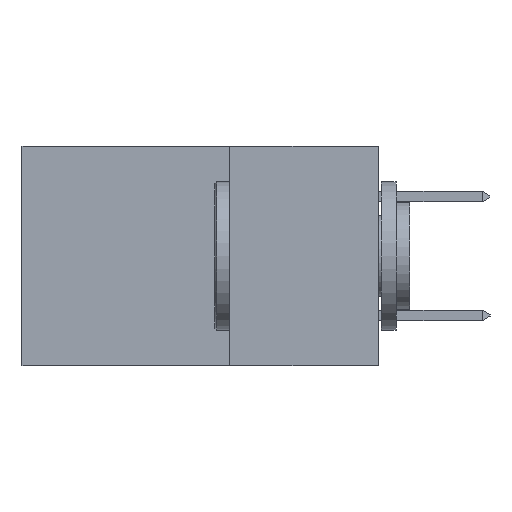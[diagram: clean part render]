
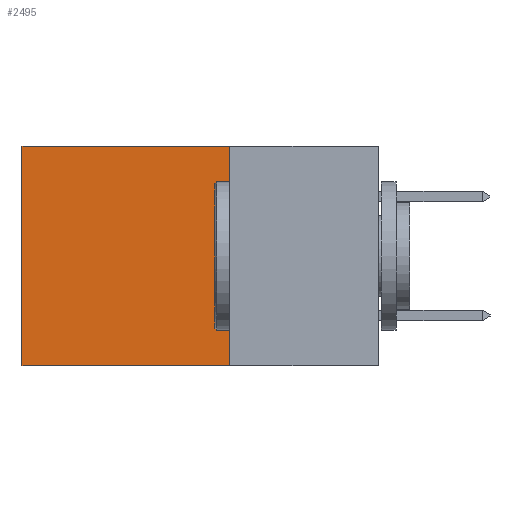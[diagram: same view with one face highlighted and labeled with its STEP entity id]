
A CAD part, left-side view. The second image highlights one B-rep face of the part: STEP entity #2495.
In plain terms, the highlighted planar face has unit normal (-1, 0, 0).
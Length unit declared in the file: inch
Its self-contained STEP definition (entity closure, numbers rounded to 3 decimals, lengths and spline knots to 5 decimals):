
#121 = VERTEX_POINT ( 'NONE', #280 ) ;
#280 = CARTESIAN_POINT ( 'NONE',  ( 0.2615, 0.6, -0.37 ) ) ;
#364 = CARTESIAN_POINT ( 'NONE',  ( 0.2615, 0.25, -0.37 ) ) ;
#738 = FACE_OUTER_BOUND ( 'NONE', #6345, .T. ) ;
#921 = DIRECTION ( 'NONE',  ( 0., 1., 0. ) ) ;
#1114 = ORIENTED_EDGE ( 'NONE', *, *, #1243, .F. ) ;
#1243 = EDGE_CURVE ( 'NONE', #9178, #2398, #4996, .T. ) ;
#1311 = VECTOR ( 'NONE', #1403, 39.37008 ) ;
#1403 = DIRECTION ( 'NONE',  ( 0., 0., -1. ) ) ;
#1466 = CARTESIAN_POINT ( 'NONE',  ( 0.2615, 0.6, -0.37 ) ) ;
#1481 = DIRECTION ( 'NONE',  ( 0., 0., -1. ) ) ;
#2011 = CARTESIAN_POINT ( 'NONE',  ( 0.2615, 0.25, 0. ) ) ;
#2398 = VERTEX_POINT ( 'NONE', #7654 ) ;
#2411 = ORIENTED_EDGE ( 'NONE', *, *, #7054, .T. ) ;
#2495 = ADVANCED_FACE ( 'NONE', ( #738 ), #4342, .F. ) ;
#2580 = ORIENTED_EDGE ( 'NONE', *, *, #2850, .T. ) ;
#2850 = EDGE_CURVE ( 'NONE', #9178, #6751, #3433, .T. ) ;
#3433 = LINE ( 'NONE', #5649, #6733 ) ;
#3653 = CARTESIAN_POINT ( 'NONE',  ( 0.2615, 0.6, 0. ) ) ;
#4156 = LINE ( 'NONE', #1466, #5811 ) ;
#4342 = PLANE ( 'NONE',  #7334 ) ;
#4824 = DIRECTION ( 'NONE',  ( 0., 0., -1. ) ) ;
#4872 = CARTESIAN_POINT ( 'NONE',  ( 0.2615, 0.25, -0.37 ) ) ;
#4996 = LINE ( 'NONE', #6114, #1311 ) ;
#5649 = CARTESIAN_POINT ( 'NONE',  ( 0.2615, 0.25, 0. ) ) ;
#5811 = VECTOR ( 'NONE', #1481, 39.37008 ) ;
#6114 = CARTESIAN_POINT ( 'NONE',  ( 0.2615, 0.25, -0.37 ) ) ;
#6345 = EDGE_LOOP ( 'NONE', ( #2411, #6411, #1114, #2580 ) ) ;
#6411 = ORIENTED_EDGE ( 'NONE', *, *, #9090, .F. ) ;
#6733 = VECTOR ( 'NONE', #921, 39.37008 ) ;
#6751 = VERTEX_POINT ( 'NONE', #3653 ) ;
#7044 = LINE ( 'NONE', #364, #7489 ) ;
#7054 = EDGE_CURVE ( 'NONE', #6751, #121, #4156, .T. ) ;
#7334 = AXIS2_PLACEMENT_3D ( 'NONE', #4872, #7814, #4824 ) ;
#7489 = VECTOR ( 'NONE', #8294, 39.37008 ) ;
#7654 = CARTESIAN_POINT ( 'NONE',  ( 0.2615, 0.25, -0.37 ) ) ;
#7814 = DIRECTION ( 'NONE',  ( 1., 0., 0. ) ) ;
#8294 = DIRECTION ( 'NONE',  ( 0., 1., 0. ) ) ;
#9090 = EDGE_CURVE ( 'NONE', #2398, #121, #7044, .T. ) ;
#9178 = VERTEX_POINT ( 'NONE', #2011 ) ;
